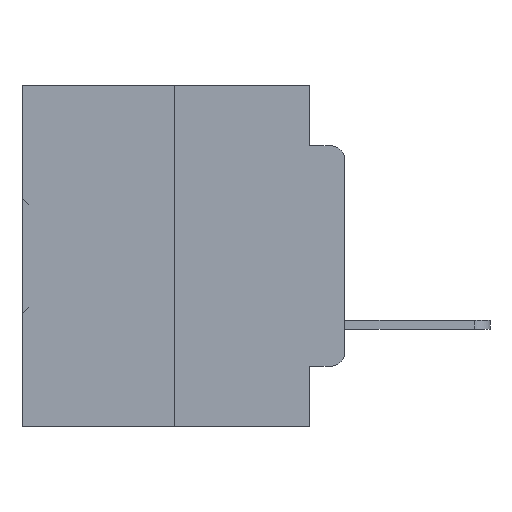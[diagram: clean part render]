
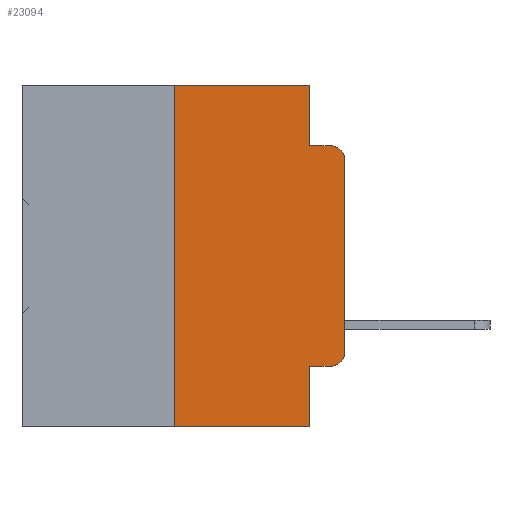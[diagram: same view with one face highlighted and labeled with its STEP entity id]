
A CAD part, left-side view. The second image highlights one B-rep face of the part: STEP entity #23094.
In plain terms, the highlighted planar face has unit normal (-1, 0, 0).
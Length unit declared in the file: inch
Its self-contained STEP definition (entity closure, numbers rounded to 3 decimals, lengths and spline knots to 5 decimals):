
#175 = VERTEX_POINT ( 'NONE', #34823 ) ;
#450 = EDGE_CURVE ( 'NONE', #2734, #175, #13490, .T. ) ;
#456 = EDGE_CURVE ( 'NONE', #13492, #2734, #27100, .T. ) ;
#525 = CARTESIAN_POINT ( 'NONE',  ( 0., 0.051, 0. ) ) ;
#696 = EDGE_CURVE ( 'NONE', #13492, #15163, #31850, .T. ) ;
#741 = LINE ( 'NONE', #7934, #29739 ) ;
#755 = EDGE_CURVE ( 'NONE', #14816, #22248, #2359, .T. ) ;
#760 = CARTESIAN_POINT ( 'NONE',  ( 0., 0.051, -0.0885 ) ) ;
#827 = EDGE_CURVE ( 'NONE', #20958, #16106, #20873, .T. ) ;
#993 = EDGE_CURVE ( 'NONE', #16106, #24554, #14781, .T. ) ;
#1346 = EDGE_CURVE ( 'NONE', #23088, #24554, #18252, .T. ) ;
#1404 = DIRECTION ( 'NONE',  ( 0., 0., 1. ) ) ;
#1408 = EDGE_CURVE ( 'NONE', #175, #23088, #7837, .T. ) ;
#2359 = LINE ( 'NONE', #31728, #8383 ) ;
#2734 = VERTEX_POINT ( 'NONE', #8721 ) ;
#3657 = ORIENTED_EDGE ( 'NONE', *, *, #1408, .T. ) ;
#5586 = ORIENTED_EDGE ( 'NONE', *, *, #1346, .T. ) ;
#6463 = CARTESIAN_POINT ( 'NONE',  ( 0., 0.25, -0.5 ) ) ;
#6903 = VECTOR ( 'NONE', #26944, 39.37008 ) ;
#6938 = VECTOR ( 'NONE', #13340, 39.37008 ) ;
#7340 = ORIENTED_EDGE ( 'NONE', *, *, #993, .F. ) ;
#7837 = LINE ( 'NONE', #34095, #6903 ) ;
#7934 = CARTESIAN_POINT ( 'NONE',  ( 0., 0.473, -0.5 ) ) ;
#7969 = CARTESIAN_POINT ( 'NONE',  ( 0., 0.051, -0.5 ) ) ;
#8265 = ORIENTED_EDGE ( 'NONE', *, *, #827, .F. ) ;
#8383 = VECTOR ( 'NONE', #1404, 39.37008 ) ;
#8721 = CARTESIAN_POINT ( 'NONE',  ( 0., 0.02, -0.4115 ) ) ;
#9415 = AXIS2_PLACEMENT_3D ( 'NONE', #10296, #27659, #18066 ) ;
#9539 = ORIENTED_EDGE ( 'NONE', *, *, #30195, .F. ) ;
#10296 = CARTESIAN_POINT ( 'NONE',  ( 0., 0.02, -0.1085 ) ) ;
#10434 = ORIENTED_EDGE ( 'NONE', *, *, #755, .F. ) ;
#12032 = ORIENTED_EDGE ( 'NONE', *, *, #13923, .T. ) ;
#12572 = VECTOR ( 'NONE', #24692, 39.37008 ) ;
#13340 = DIRECTION ( 'NONE',  ( 0., -1., 0. ) ) ;
#13490 = CIRCLE ( 'NONE', #35599, 0.02 ) ;
#13492 = VERTEX_POINT ( 'NONE', #35551 ) ;
#13702 = CARTESIAN_POINT ( 'NONE',  ( 0., 0.051, 0. ) ) ;
#13923 = EDGE_CURVE ( 'NONE', #14816, #15163, #741, .T. ) ;
#14178 = ORIENTED_EDGE ( 'NONE', *, *, #696, .F. ) ;
#14781 = LINE ( 'NONE', #760, #6938 ) ;
#14816 = VERTEX_POINT ( 'NONE', #6463 ) ;
#15163 = VERTEX_POINT ( 'NONE', #7969 ) ;
#15291 = CARTESIAN_POINT ( 'NONE',  ( 0., 0.051, 0. ) ) ;
#16106 = VERTEX_POINT ( 'NONE', #16744 ) ;
#16252 = DIRECTION ( 'NONE',  ( 1., 0., 0. ) ) ;
#16744 = CARTESIAN_POINT ( 'NONE',  ( 0., 0.051, -0.0885 ) ) ;
#17217 = ORIENTED_EDGE ( 'NONE', *, *, #456, .T. ) ;
#18066 = DIRECTION ( 'NONE',  ( 0., 0., -1. ) ) ;
#18252 = CIRCLE ( 'NONE', #9415, 0.02 ) ;
#19511 = ORIENTED_EDGE ( 'NONE', *, *, #450, .T. ) ;
#19705 = DIRECTION ( 'NONE',  ( 0., 0., -1. ) ) ;
#20077 = EDGE_LOOP ( 'NONE', ( #3657, #5586, #7340, #8265, #9539, #10434, #12032, #14178, #17217, #19511 ) ) ;
#20873 = LINE ( 'NONE', #13702, #33824 ) ;
#20958 = VERTEX_POINT ( 'NONE', #525 ) ;
#22248 = VERTEX_POINT ( 'NONE', #28397 ) ;
#23088 = VERTEX_POINT ( 'NONE', #26870 ) ;
#23094 = ADVANCED_FACE ( 'NONE', ( #31178 ), #34540, .F. ) ;
#24243 = CARTESIAN_POINT ( 'NONE',  ( 0., 0.473, 0. ) ) ;
#24365 = DIRECTION ( 'NONE',  ( 0., -1., 0. ) ) ;
#24554 = VERTEX_POINT ( 'NONE', #27338 ) ;
#24692 = DIRECTION ( 'NONE',  ( 0., -1., 0. ) ) ;
#24708 = DIRECTION ( 'NONE',  ( 0., 0., -1. ) ) ;
#25020 = VECTOR ( 'NONE', #24708, 39.37008 ) ;
#25347 = DIRECTION ( 'NONE',  ( 0., 0., -1. ) ) ;
#26476 = CARTESIAN_POINT ( 'NONE',  ( 0., 0.02, -0.3915 ) ) ;
#26739 = DIRECTION ( 'NONE',  ( -1., 0., 0. ) ) ;
#26870 = CARTESIAN_POINT ( 'NONE',  ( 0., 0., -0.1085 ) ) ;
#26944 = DIRECTION ( 'NONE',  ( 0., 0., 1. ) ) ;
#27100 = LINE ( 'NONE', #35391, #12572 ) ;
#27338 = CARTESIAN_POINT ( 'NONE',  ( 0., 0.02, -0.0885 ) ) ;
#27659 = DIRECTION ( 'NONE',  ( -1., 0., 0. ) ) ;
#27982 = VECTOR ( 'NONE', #24365, 39.37008 ) ;
#28397 = CARTESIAN_POINT ( 'NONE',  ( 0., 0.25, 0. ) ) ;
#28676 = AXIS2_PLACEMENT_3D ( 'NONE', #32090, #16252, #34647 ) ;
#29739 = VECTOR ( 'NONE', #30062, 39.37008 ) ;
#30062 = DIRECTION ( 'NONE',  ( 0., -1., 0. ) ) ;
#30195 = EDGE_CURVE ( 'NONE', #22248, #20958, #35529, .T. ) ;
#31178 = FACE_OUTER_BOUND ( 'NONE', #20077, .T. ) ;
#31728 = CARTESIAN_POINT ( 'NONE',  ( 0., 0.25, 0. ) ) ;
#31850 = LINE ( 'NONE', #15291, #25020 ) ;
#32090 = CARTESIAN_POINT ( 'NONE',  ( 0., 0.473, 0. ) ) ;
#33824 = VECTOR ( 'NONE', #19705, 39.37008 ) ;
#34095 = CARTESIAN_POINT ( 'NONE',  ( 0., 0., 0. ) ) ;
#34540 = PLANE ( 'NONE',  #28676 ) ;
#34647 = DIRECTION ( 'NONE',  ( 0., 0., -1. ) ) ;
#34823 = CARTESIAN_POINT ( 'NONE',  ( 0., 0., -0.3915 ) ) ;
#35391 = CARTESIAN_POINT ( 'NONE',  ( 0., 0.051, -0.4115 ) ) ;
#35529 = LINE ( 'NONE', #24243, #27982 ) ;
#35551 = CARTESIAN_POINT ( 'NONE',  ( 0., 0.051, -0.4115 ) ) ;
#35599 = AXIS2_PLACEMENT_3D ( 'NONE', #26476, #26739, #25347 ) ;
